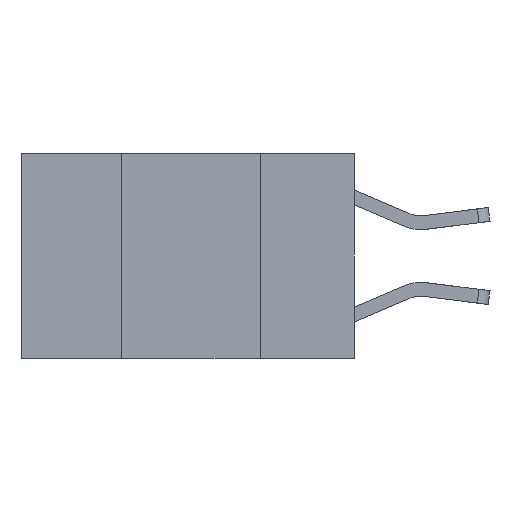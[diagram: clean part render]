
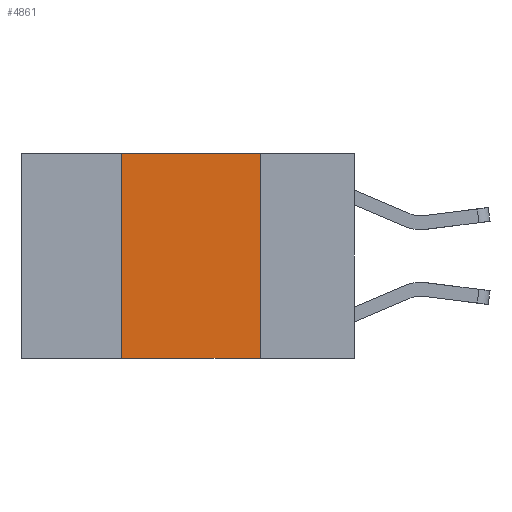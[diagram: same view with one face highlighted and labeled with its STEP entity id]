
A CAD part, left-side view. The second image highlights one B-rep face of the part: STEP entity #4861.
In plain terms, the highlighted planar face has unit normal (-1, 0, 0).
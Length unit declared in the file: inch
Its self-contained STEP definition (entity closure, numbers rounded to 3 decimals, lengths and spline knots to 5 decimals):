
#248 = AXIS2_PLACEMENT_3D ( 'NONE', #2969, #7497, #4103 ) ;
#280 = LINE ( 'NONE', #5422, #422 ) ;
#422 = VECTOR ( 'NONE', #10546, 39.37008 ) ;
#805 = LINE ( 'NONE', #3188, #10878 ) ;
#857 = DIRECTION ( 'NONE',  ( 0., -1., 0. ) ) ;
#988 = ORIENTED_EDGE ( 'NONE', *, *, #7174, .F. ) ;
#1152 = VECTOR ( 'NONE', #3475, 39.37008 ) ;
#1207 = EDGE_LOOP ( 'NONE', ( #6122, #5001, #988, #5150 ) ) ;
#1874 = VERTEX_POINT ( 'NONE', #2572 ) ;
#2161 = LINE ( 'NONE', #2889, #9847 ) ;
#2572 = CARTESIAN_POINT ( 'NONE',  ( 0., 0.42, 0. ) ) ;
#2889 = CARTESIAN_POINT ( 'NONE',  ( 0., 0.42, 0. ) ) ;
#2911 = PLANE ( 'NONE',  #248 ) ;
#2969 = CARTESIAN_POINT ( 'NONE',  ( 0., 0.6, 0. ) ) ;
#3188 = CARTESIAN_POINT ( 'NONE',  ( 0., 0.6, 0. ) ) ;
#3475 = DIRECTION ( 'NONE',  ( 0., 0., -1. ) ) ;
#3825 = FACE_OUTER_BOUND ( 'NONE', #1207, .T. ) ;
#4103 = DIRECTION ( 'NONE',  ( 0., 0., -1. ) ) ;
#4233 = CARTESIAN_POINT ( 'NONE',  ( 0., 0.17, -0.37 ) ) ;
#4279 = LINE ( 'NONE', #7779, #1152 ) ;
#4446 = CARTESIAN_POINT ( 'NONE',  ( 0., 0.17, 0. ) ) ;
#4861 = ADVANCED_FACE ( 'NONE', ( #3825 ), #2911, .F. ) ;
#5001 = ORIENTED_EDGE ( 'NONE', *, *, #6253, .F. ) ;
#5120 = EDGE_CURVE ( 'NONE', #8462, #8327, #4279, .T. ) ;
#5150 = ORIENTED_EDGE ( 'NONE', *, *, #10954, .T. ) ;
#5208 = VERTEX_POINT ( 'NONE', #8231 ) ;
#5422 = CARTESIAN_POINT ( 'NONE',  ( 0., 0.6, -0.37 ) ) ;
#5573 = DIRECTION ( 'NONE',  ( 0., 0., 1. ) ) ;
#6122 = ORIENTED_EDGE ( 'NONE', *, *, #5120, .F. ) ;
#6253 = EDGE_CURVE ( 'NONE', #1874, #8462, #805, .T. ) ;
#7174 = EDGE_CURVE ( 'NONE', #5208, #1874, #2161, .T. ) ;
#7497 = DIRECTION ( 'NONE',  ( 1., 0., 0. ) ) ;
#7779 = CARTESIAN_POINT ( 'NONE',  ( 0., 0.17, 0. ) ) ;
#8231 = CARTESIAN_POINT ( 'NONE',  ( 0., 0.42, -0.37 ) ) ;
#8327 = VERTEX_POINT ( 'NONE', #4233 ) ;
#8462 = VERTEX_POINT ( 'NONE', #4446 ) ;
#9847 = VECTOR ( 'NONE', #5573, 39.37008 ) ;
#10546 = DIRECTION ( 'NONE',  ( 0., -1., 0. ) ) ;
#10878 = VECTOR ( 'NONE', #857, 39.37008 ) ;
#10954 = EDGE_CURVE ( 'NONE', #5208, #8327, #280, .T. ) ;
